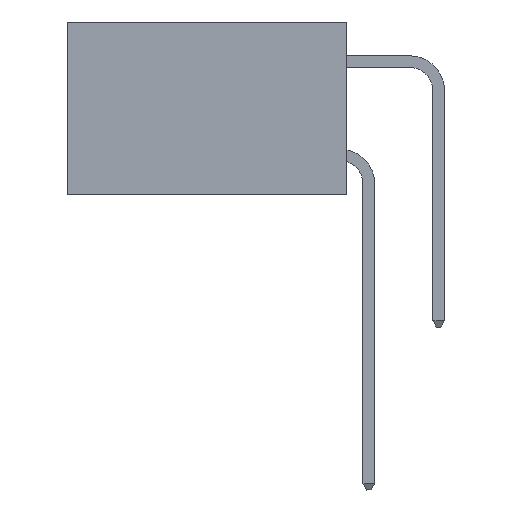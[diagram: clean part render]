
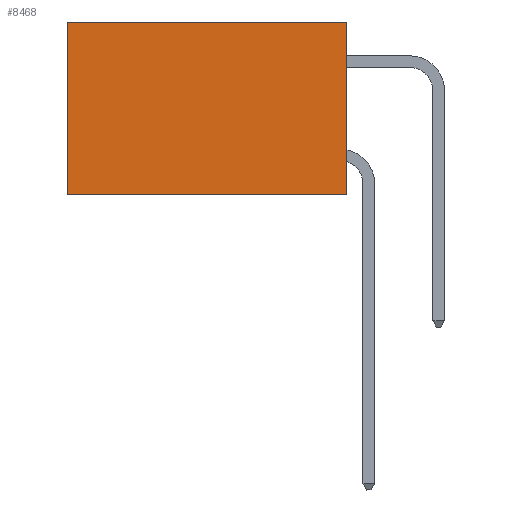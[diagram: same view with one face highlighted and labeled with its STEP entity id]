
A CAD part, left-side view. The second image highlights one B-rep face of the part: STEP entity #8468.
In plain terms, the highlighted planar face has unit normal (-1, 0, 0).
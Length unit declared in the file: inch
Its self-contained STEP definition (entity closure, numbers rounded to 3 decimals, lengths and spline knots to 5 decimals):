
#513 = DIRECTION ( 'NONE',  ( 1., 0., 0. ) ) ;
#886 = ORIENTED_EDGE ( 'NONE', *, *, #10435, .T. ) ;
#1164 = DIRECTION ( 'NONE',  ( 0., 0., -1. ) ) ;
#1320 = CARTESIAN_POINT ( 'NONE',  ( 0.2875, 0., 0. ) ) ;
#1544 = CARTESIAN_POINT ( 'NONE',  ( 0.2875, 0., 0. ) ) ;
#1782 = VERTEX_POINT ( 'NONE', #8848 ) ;
#2137 = ORIENTED_EDGE ( 'NONE', *, *, #6090, .F. ) ;
#2463 = LINE ( 'NONE', #7771, #12578 ) ;
#3269 = VERTEX_POINT ( 'NONE', #5510 ) ;
#3458 = CARTESIAN_POINT ( 'NONE',  ( 0.2875, 0.6, 0. ) ) ;
#3729 = DIRECTION ( 'NONE',  ( 0., 1., 0. ) ) ;
#3919 = VECTOR ( 'NONE', #11308, 39.37008 ) ;
#4873 = PLANE ( 'NONE',  #8853 ) ;
#5510 = CARTESIAN_POINT ( 'NONE',  ( 0.2875, 0., -0.37 ) ) ;
#5548 = CARTESIAN_POINT ( 'NONE',  ( 0.2875, 0., 0. ) ) ;
#6090 = EDGE_CURVE ( 'NONE', #6701, #3269, #9755, .T. ) ;
#6309 = ORIENTED_EDGE ( 'NONE', *, *, #7640, .T. ) ;
#6617 = LINE ( 'NONE', #5548, #3919 ) ;
#6701 = VERTEX_POINT ( 'NONE', #9199 ) ;
#7194 = VERTEX_POINT ( 'NONE', #3458 ) ;
#7239 = DIRECTION ( 'NONE',  ( 0., 0., -1. ) ) ;
#7275 = VECTOR ( 'NONE', #1164, 39.37008 ) ;
#7640 = EDGE_CURVE ( 'NONE', #7194, #1782, #9862, .T. ) ;
#7771 = CARTESIAN_POINT ( 'NONE',  ( 0.2875, 0., -0.37 ) ) ;
#7861 = DIRECTION ( 'NONE',  ( 0., 0., -1. ) ) ;
#8450 = CARTESIAN_POINT ( 'NONE',  ( 0.2875, 0.6, 0. ) ) ;
#8468 = ADVANCED_FACE ( 'NONE', ( #12475 ), #4873, .F. ) ;
#8848 = CARTESIAN_POINT ( 'NONE',  ( 0.2875, 0.6, -0.37 ) ) ;
#8853 = AXIS2_PLACEMENT_3D ( 'NONE', #1544, #513, #7861 ) ;
#8922 = ORIENTED_EDGE ( 'NONE', *, *, #10568, .F. ) ;
#9199 = CARTESIAN_POINT ( 'NONE',  ( 0.2875, 0., 0. ) ) ;
#9446 = VECTOR ( 'NONE', #7239, 39.37008 ) ;
#9755 = LINE ( 'NONE', #1320, #9446 ) ;
#9862 = LINE ( 'NONE', #8450, #7275 ) ;
#10435 = EDGE_CURVE ( 'NONE', #6701, #7194, #6617, .T. ) ;
#10568 = EDGE_CURVE ( 'NONE', #3269, #1782, #2463, .T. ) ;
#11308 = DIRECTION ( 'NONE',  ( 0., 1., 0. ) ) ;
#12288 = EDGE_LOOP ( 'NONE', ( #6309, #8922, #2137, #886 ) ) ;
#12475 = FACE_OUTER_BOUND ( 'NONE', #12288, .T. ) ;
#12578 = VECTOR ( 'NONE', #3729, 39.37008 ) ;
